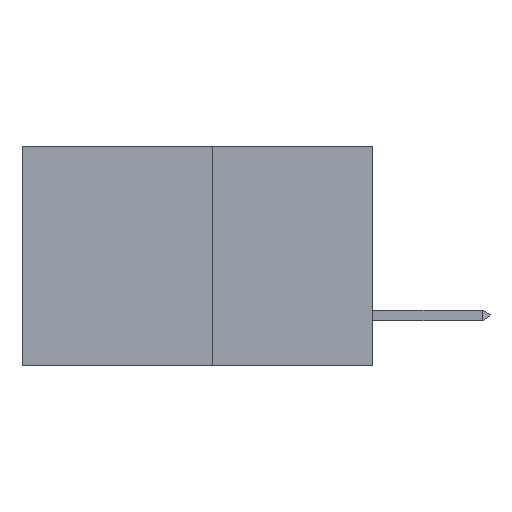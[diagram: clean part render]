
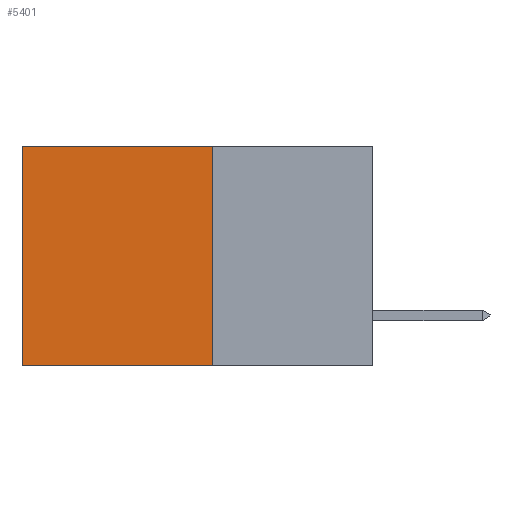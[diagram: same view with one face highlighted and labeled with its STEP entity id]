
A CAD part, left-side view. The second image highlights one B-rep face of the part: STEP entity #5401.
In plain terms, the highlighted planar face has unit normal (-1, 0, 0).
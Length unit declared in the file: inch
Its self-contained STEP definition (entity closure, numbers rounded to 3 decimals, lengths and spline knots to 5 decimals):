
#84 = VERTEX_POINT ( 'NONE', #7025 ) ;
#327 = DIRECTION ( 'NONE',  ( 0., 0., -1. ) ) ;
#526 = EDGE_CURVE ( 'NONE', #6140, #8639, #3509, .T. ) ;
#645 = FACE_OUTER_BOUND ( 'NONE', #3879, .T. ) ;
#1382 = VERTEX_POINT ( 'NONE', #7641 ) ;
#3103 = DIRECTION ( 'NONE',  ( 0., 1., 0. ) ) ;
#3131 = CARTESIAN_POINT ( 'NONE',  ( 0.277, 0.27, -0.37 ) ) ;
#3509 = LINE ( 'NONE', #7588, #10091 ) ;
#3526 = VECTOR ( 'NONE', #327, 39.37008 ) ;
#3879 = EDGE_LOOP ( 'NONE', ( #9800, #5474, #7731, #10068 ) ) ;
#4567 = LINE ( 'NONE', #3131, #8890 ) ;
#4660 = DIRECTION ( 'NONE',  ( 0., 1., 0. ) ) ;
#4720 = VECTOR ( 'NONE', #4660, 39.37008 ) ;
#5068 = DIRECTION ( 'NONE',  ( 1., 0., 0. ) ) ;
#5401 = ADVANCED_FACE ( 'NONE', ( #645 ), #7126, .F. ) ;
#5474 = ORIENTED_EDGE ( 'NONE', *, *, #6052, .F. ) ;
#5484 = CARTESIAN_POINT ( 'NONE',  ( 0.277, 0.27, 0. ) ) ;
#5839 = EDGE_CURVE ( 'NONE', #84, #1382, #10373, .T. ) ;
#6052 = EDGE_CURVE ( 'NONE', #8639, #1382, #4567, .T. ) ;
#6140 = VERTEX_POINT ( 'NONE', #6845 ) ;
#6343 = CARTESIAN_POINT ( 'NONE',  ( 0.277, 0.27, -0.37 ) ) ;
#6388 = DIRECTION ( 'NONE',  ( 0., 0., -1. ) ) ;
#6522 = AXIS2_PLACEMENT_3D ( 'NONE', #6343, #5068, #6388 ) ;
#6845 = CARTESIAN_POINT ( 'NONE',  ( 0.277, 0.27, 0. ) ) ;
#6957 = LINE ( 'NONE', #5484, #4720 ) ;
#7025 = CARTESIAN_POINT ( 'NONE',  ( 0.277, 0.59, 0. ) ) ;
#7126 = PLANE ( 'NONE',  #6522 ) ;
#7588 = CARTESIAN_POINT ( 'NONE',  ( 0.277, 0.27, -0.37 ) ) ;
#7641 = CARTESIAN_POINT ( 'NONE',  ( 0.277, 0.59, -0.37 ) ) ;
#7731 = ORIENTED_EDGE ( 'NONE', *, *, #526, .F. ) ;
#8639 = VERTEX_POINT ( 'NONE', #11028 ) ;
#8890 = VECTOR ( 'NONE', #3103, 39.37008 ) ;
#9120 = EDGE_CURVE ( 'NONE', #6140, #84, #6957, .T. ) ;
#9800 = ORIENTED_EDGE ( 'NONE', *, *, #5839, .T. ) ;
#10068 = ORIENTED_EDGE ( 'NONE', *, *, #9120, .T. ) ;
#10085 = DIRECTION ( 'NONE',  ( 0., 0., -1. ) ) ;
#10091 = VECTOR ( 'NONE', #10085, 39.37008 ) ;
#10373 = LINE ( 'NONE', #11182, #3526 ) ;
#11028 = CARTESIAN_POINT ( 'NONE',  ( 0.277, 0.27, -0.37 ) ) ;
#11182 = CARTESIAN_POINT ( 'NONE',  ( 0.277, 0.59, -0.37 ) ) ;
